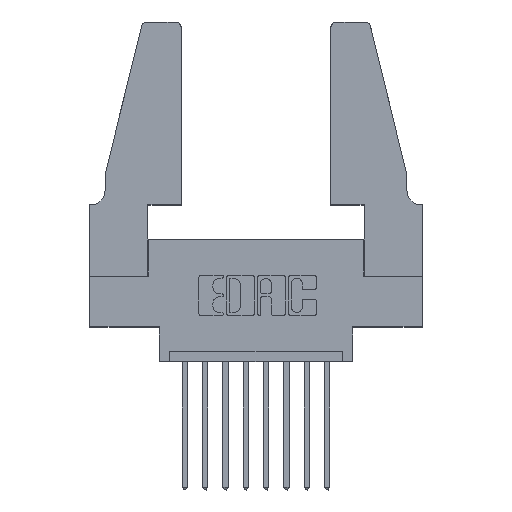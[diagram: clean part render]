
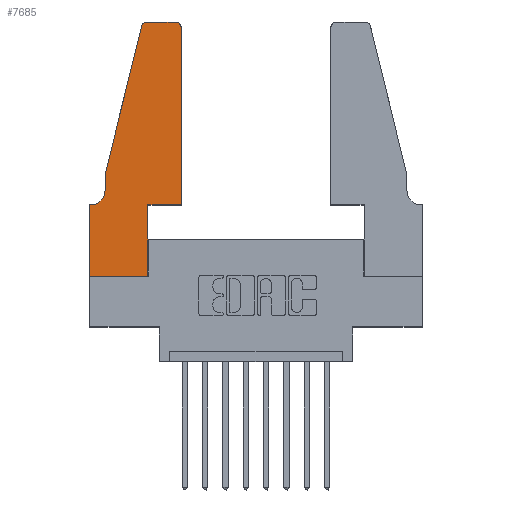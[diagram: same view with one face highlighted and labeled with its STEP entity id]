
A CAD part, top view. The second image highlights one B-rep face of the part: STEP entity #7685.
In plain terms, the highlighted planar face has unit normal (0, 0, 1).
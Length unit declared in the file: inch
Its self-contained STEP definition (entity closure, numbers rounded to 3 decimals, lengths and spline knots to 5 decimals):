
#89 = DIRECTION ( 'NONE',  ( 0., 0., -1. ) ) ;
#115 = LINE ( 'NONE', #9981, #5060 ) ;
#247 = DIRECTION ( 'NONE',  ( -1., 0., 0. ) ) ;
#319 = DIRECTION ( 'NONE',  ( 0., 1., 0. ) ) ;
#387 = ORIENTED_EDGE ( 'NONE', *, *, #5496, .T. ) ;
#396 = CARTESIAN_POINT ( 'NONE',  ( 0.284, 1.22, 0.37 ) ) ;
#411 = VECTOR ( 'NONE', #4490, 39.37008 ) ;
#677 = DIRECTION ( 'NONE',  ( 1., 0., 0. ) ) ;
#733 = FACE_OUTER_BOUND ( 'NONE', #9362, .T. ) ;
#1077 = CARTESIAN_POINT ( 'NONE',  ( 0.4505, 1.22, 0.37 ) ) ;
#1258 = DIRECTION ( 'NONE',  ( 0., 0., 1. ) ) ;
#1940 = CARTESIAN_POINT ( 'NONE',  ( 0.2605, 1.25, 0.37 ) ) ;
#1996 = ORIENTED_EDGE ( 'NONE', *, *, #5418, .T. ) ;
#2021 = CIRCLE ( 'NONE', #5826, 0.07 ) ;
#2141 = LINE ( 'NONE', #3757, #5218 ) ;
#2281 = LINE ( 'NONE', #6157, #12585 ) ;
#2354 = ORIENTED_EDGE ( 'NONE', *, *, #7987, .T. ) ;
#2358 = ORIENTED_EDGE ( 'NONE', *, *, #10582, .T. ) ;
#2413 = DIRECTION ( 'NONE',  ( 1., 0., 0. ) ) ;
#2465 = CARTESIAN_POINT ( 'NONE',  ( 0.0755, 0.5, 0.37 ) ) ;
#2542 = DIRECTION ( 'NONE',  ( 0., 0., 1. ) ) ;
#2580 = VERTEX_POINT ( 'NONE', #8099 ) ;
#2847 = ORIENTED_EDGE ( 'NONE', *, *, #12004, .T. ) ;
#2901 = DIRECTION ( 'NONE',  ( -1., 0., 0. ) ) ;
#2991 = ORIENTED_EDGE ( 'NONE', *, *, #9521, .T. ) ;
#3342 = LINE ( 'NONE', #2465, #411 ) ;
#3380 = CARTESIAN_POINT ( 'NONE',  ( 0.2865, 0.35, 0.37 ) ) ;
#3741 = VERTEX_POINT ( 'NONE', #9505 ) ;
#3757 = CARTESIAN_POINT ( 'NONE',  ( 0., 0., 0.37 ) ) ;
#3804 = VERTEX_POINT ( 'NONE', #6502 ) ;
#3928 = CARTESIAN_POINT ( 'NONE',  ( 0.2865, 0.35, 0.37 ) ) ;
#4173 = VERTEX_POINT ( 'NONE', #11467 ) ;
#4405 = CARTESIAN_POINT ( 'NONE',  ( 0.0755, 0.5, 0.37 ) ) ;
#4482 = CARTESIAN_POINT ( 'NONE',  ( 0.4205, 1.22, 0.37 ) ) ;
#4490 = DIRECTION ( 'NONE',  ( -0.239, -0.971, 0. ) ) ;
#4592 = ORIENTED_EDGE ( 'NONE', *, *, #12771, .T. ) ;
#4652 = VERTEX_POINT ( 'NONE', #10263 ) ;
#4902 = DIRECTION ( 'NONE',  ( 0., -1., 0. ) ) ;
#4982 = AXIS2_PLACEMENT_3D ( 'NONE', #396, #1258, #7197 ) ;
#5060 = VECTOR ( 'NONE', #4902, 39.37008 ) ;
#5218 = VECTOR ( 'NONE', #8585, 39.37008 ) ;
#5342 = PLANE ( 'NONE',  #7073 ) ;
#5415 = DIRECTION ( 'NONE',  ( 0., 1., 0. ) ) ;
#5418 = EDGE_CURVE ( 'NONE', #3804, #2580, #2021, .T. ) ;
#5450 = VERTEX_POINT ( 'NONE', #1077 ) ;
#5496 = EDGE_CURVE ( 'NONE', #6996, #4173, #10286, .T. ) ;
#5545 = VECTOR ( 'NONE', #5415, 39.37008 ) ;
#5606 = VERTEX_POINT ( 'NONE', #12193 ) ;
#5730 = EDGE_CURVE ( 'NONE', #2580, #8092, #9812, .T. ) ;
#5826 = AXIS2_PLACEMENT_3D ( 'NONE', #9032, #89, #9075 ) ;
#6109 = EDGE_CURVE ( 'NONE', #5450, #4652, #7582, .T. ) ;
#6157 = CARTESIAN_POINT ( 'NONE',  ( 0.0755, 0.5, 0.37 ) ) ;
#6502 = CARTESIAN_POINT ( 'NONE',  ( 0.0755, 0.42, 0.37 ) ) ;
#6603 = LINE ( 'NONE', #10022, #11804 ) ;
#6770 = ORIENTED_EDGE ( 'NONE', *, *, #8102, .T. ) ;
#6789 = VECTOR ( 'NONE', #247, 39.37008 ) ;
#6996 = VERTEX_POINT ( 'NONE', #10384 ) ;
#7048 = DIRECTION ( 'NONE',  ( 1., 0., 0. ) ) ;
#7073 = AXIS2_PLACEMENT_3D ( 'NONE', #11313, #8351, #2413 ) ;
#7152 = ORIENTED_EDGE ( 'NONE', *, *, #7273, .T. ) ;
#7197 = DIRECTION ( 'NONE',  ( 1., 0., 0. ) ) ;
#7196 = LINE ( 'NONE', #1940, #9912 ) ;
#7273 = EDGE_CURVE ( 'NONE', #12518, #3741, #2141, .T. ) ;
#7274 = VECTOR ( 'NONE', #319, 39.37008 ) ;
#7582 = CIRCLE ( 'NONE', #7905, 0.03 ) ;
#7685 = ADVANCED_FACE ( 'NONE', ( #733 ), #5342, .T. ) ;
#7905 = AXIS2_PLACEMENT_3D ( 'NONE', #4482, #2542, #677 ) ;
#7987 = EDGE_CURVE ( 'NONE', #4652, #6996, #7196, .T. ) ;
#8081 = EDGE_CURVE ( 'NONE', #10028, #5606, #6603, .T. ) ;
#8092 = VERTEX_POINT ( 'NONE', #11051 ) ;
#8099 = CARTESIAN_POINT ( 'NONE',  ( 0.0055, 0.35, 0.37 ) ) ;
#8102 = EDGE_CURVE ( 'NONE', #8092, #12518, #115, .T. ) ;
#8212 = ORIENTED_EDGE ( 'NONE', *, *, #6109, .T. ) ;
#8252 = ORIENTED_EDGE ( 'NONE', *, *, #8081, .T. ) ;
#8351 = DIRECTION ( 'NONE',  ( 0., 0., 1. ) ) ;
#8585 = DIRECTION ( 'NONE',  ( 1., 0., 0. ) ) ;
#8820 = LINE ( 'NONE', #3380, #5545 ) ;
#9032 = CARTESIAN_POINT ( 'NONE',  ( 0.0055, 0.42, 0.37 ) ) ;
#9075 = DIRECTION ( 'NONE',  ( -1., 0., 0. ) ) ;
#9362 = EDGE_LOOP ( 'NONE', ( #2354, #387, #4592, #2847, #1996, #11202, #6770, #7152, #2358, #8252, #2991, #8212 ) ) ;
#9505 = CARTESIAN_POINT ( 'NONE',  ( 0.2865, 0., 0.37 ) ) ;
#9521 = EDGE_CURVE ( 'NONE', #5606, #5450, #11552, .T. ) ;
#9812 = LINE ( 'NONE', #10033, #6789 ) ;
#9912 = VECTOR ( 'NONE', #2901, 39.37008 ) ;
#9981 = CARTESIAN_POINT ( 'NONE',  ( 0., 0., 0.37 ) ) ;
#10022 = CARTESIAN_POINT ( 'NONE',  ( 0.4505, 0.35, 0.37 ) ) ;
#10028 = VERTEX_POINT ( 'NONE', #3928 ) ;
#10033 = CARTESIAN_POINT ( 'NONE',  ( 0.0755, 0.35, 0.37 ) ) ;
#10057 = DIRECTION ( 'NONE',  ( 0., -1., 0. ) ) ;
#10263 = CARTESIAN_POINT ( 'NONE',  ( 0.4205, 1.25, 0.37 ) ) ;
#10286 = CIRCLE ( 'NONE', #4982, 0.03 ) ;
#10384 = CARTESIAN_POINT ( 'NONE',  ( 0.284, 1.25, 0.37 ) ) ;
#10582 = EDGE_CURVE ( 'NONE', #3741, #10028, #8820, .T. ) ;
#11020 = VERTEX_POINT ( 'NONE', #4405 ) ;
#11051 = CARTESIAN_POINT ( 'NONE',  ( 0., 0.35, 0.37 ) ) ;
#11202 = ORIENTED_EDGE ( 'NONE', *, *, #5730, .T. ) ;
#11313 = CARTESIAN_POINT ( 'NONE',  ( 0., 0.35, 0.37 ) ) ;
#11343 = CARTESIAN_POINT ( 'NONE',  ( 0.4505, 0.35, 0.37 ) ) ;
#11447 = CARTESIAN_POINT ( 'NONE',  ( 0., 0., 0.37 ) ) ;
#11467 = CARTESIAN_POINT ( 'NONE',  ( 0.25487, 1.22718, 0.37 ) ) ;
#11552 = LINE ( 'NONE', #11343, #7274 ) ;
#11804 = VECTOR ( 'NONE', #7048, 39.37008 ) ;
#12004 = EDGE_CURVE ( 'NONE', #11020, #3804, #2281, .T. ) ;
#12193 = CARTESIAN_POINT ( 'NONE',  ( 0.4505, 0.35, 0.37 ) ) ;
#12518 = VERTEX_POINT ( 'NONE', #11447 ) ;
#12585 = VECTOR ( 'NONE', #10057, 39.37008 ) ;
#12771 = EDGE_CURVE ( 'NONE', #4173, #11020, #3342, .T. ) ;
